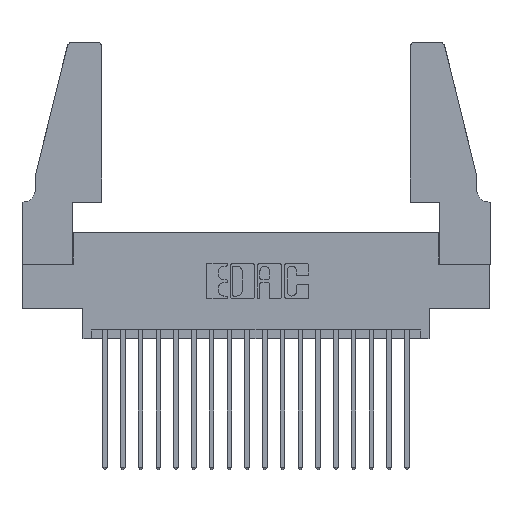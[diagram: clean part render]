
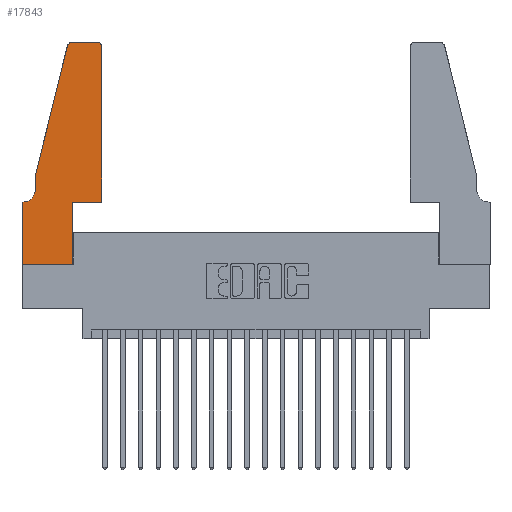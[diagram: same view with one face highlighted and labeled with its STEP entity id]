
A CAD part, top view. The second image highlights one B-rep face of the part: STEP entity #17843.
In plain terms, the highlighted planar face has unit normal (0, 0, 1).
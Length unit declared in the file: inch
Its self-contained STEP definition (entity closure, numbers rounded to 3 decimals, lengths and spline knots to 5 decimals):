
#2 = CARTESIAN_POINT ( 'NONE',  ( 0.0755, 0.5, 0.37 ) ) ;
#9 = DIRECTION ( 'NONE',  ( 0., 1., 0. ) ) ;
#520 = CARTESIAN_POINT ( 'NONE',  ( 0.4505, 0.35, 0.37 ) ) ;
#536 = ORIENTED_EDGE ( 'NONE', *, *, #3863, .T. ) ;
#631 = CARTESIAN_POINT ( 'NONE',  ( 0.4505, 0.35, 0.37 ) ) ;
#788 = DIRECTION ( 'NONE',  ( 0., 0., 1. ) ) ;
#1027 = LINE ( 'NONE', #520, #5373 ) ;
#1631 = VERTEX_POINT ( 'NONE', #18166 ) ;
#1721 = CARTESIAN_POINT ( 'NONE',  ( 0.0755, 0.42, 0.37 ) ) ;
#1843 = ORIENTED_EDGE ( 'NONE', *, *, #14942, .T. ) ;
#2127 = FACE_OUTER_BOUND ( 'NONE', #16101, .T. ) ;
#2367 = ORIENTED_EDGE ( 'NONE', *, *, #18949, .T. ) ;
#2944 = VERTEX_POINT ( 'NONE', #4091 ) ;
#3364 = VECTOR ( 'NONE', #5331, 39.37008 ) ;
#3475 = LINE ( 'NONE', #19083, #18404 ) ;
#3617 = EDGE_CURVE ( 'NONE', #4269, #6667, #7721, .T. ) ;
#3683 = DIRECTION ( 'NONE',  ( 0., 0., 1. ) ) ;
#3755 = CARTESIAN_POINT ( 'NONE',  ( 0.0755, 0.35, 0.37 ) ) ;
#3863 = EDGE_CURVE ( 'NONE', #18219, #6920, #7946, .T. ) ;
#3921 = ORIENTED_EDGE ( 'NONE', *, *, #6790, .T. ) ;
#3951 = EDGE_CURVE ( 'NONE', #12630, #5496, #13913, .T. ) ;
#4091 = CARTESIAN_POINT ( 'NONE',  ( 0.2865, 0.35, 0.37 ) ) ;
#4269 = VERTEX_POINT ( 'NONE', #14150 ) ;
#4566 = CARTESIAN_POINT ( 'NONE',  ( 0.4505, 1.22, 0.37 ) ) ;
#4882 = AXIS2_PLACEMENT_3D ( 'NONE', #5209, #3683, #14133 ) ;
#5209 = CARTESIAN_POINT ( 'NONE',  ( 0., 0.35, 0.37 ) ) ;
#5331 = DIRECTION ( 'NONE',  ( -1., 0., 0. ) ) ;
#5355 = LINE ( 'NONE', #2, #16715 ) ;
#5373 = VECTOR ( 'NONE', #11367, 39.37008 ) ;
#5496 = VERTEX_POINT ( 'NONE', #8089 ) ;
#5826 = EDGE_CURVE ( 'NONE', #6920, #4269, #3475, .T. ) ;
#6178 = AXIS2_PLACEMENT_3D ( 'NONE', #10851, #15654, #16074 ) ;
#6278 = CARTESIAN_POINT ( 'NONE',  ( 0., 0., 0.37 ) ) ;
#6507 = CARTESIAN_POINT ( 'NONE',  ( 0.0055, 0.42, 0.37 ) ) ;
#6520 = VERTEX_POINT ( 'NONE', #13166 ) ;
#6667 = VERTEX_POINT ( 'NONE', #7659 ) ;
#6790 = EDGE_CURVE ( 'NONE', #5496, #2944, #17440, .T. ) ;
#6920 = VERTEX_POINT ( 'NONE', #15602 ) ;
#7625 = CIRCLE ( 'NONE', #16728, 0.07 ) ;
#7659 = CARTESIAN_POINT ( 'NONE',  ( 0.25487, 1.22718, 0.37 ) ) ;
#7721 = CIRCLE ( 'NONE', #6178, 0.03 ) ;
#7946 = CIRCLE ( 'NONE', #16095, 0.03 ) ;
#8030 = DIRECTION ( 'NONE',  ( -1., 0., 0. ) ) ;
#8089 = CARTESIAN_POINT ( 'NONE',  ( 0.2865, 0., 0.37 ) ) ;
#8782 = DIRECTION ( 'NONE',  ( -1., 0., 0. ) ) ;
#9152 = ORIENTED_EDGE ( 'NONE', *, *, #5826, .T. ) ;
#9275 = CARTESIAN_POINT ( 'NONE',  ( 0.0055, 0.35, 0.37 ) ) ;
#10003 = DIRECTION ( 'NONE',  ( 0., 1., 0. ) ) ;
#10021 = VECTOR ( 'NONE', #19143, 39.37008 ) ;
#10087 = CARTESIAN_POINT ( 'NONE',  ( 0., 0., 0.37 ) ) ;
#10132 = CARTESIAN_POINT ( 'NONE',  ( 0.4205, 1.22, 0.37 ) ) ;
#10447 = EDGE_CURVE ( 'NONE', #17723, #12244, #7625, .T. ) ;
#10533 = ORIENTED_EDGE ( 'NONE', *, *, #10447, .T. ) ;
#10851 = CARTESIAN_POINT ( 'NONE',  ( 0.284, 1.22, 0.37 ) ) ;
#11367 = DIRECTION ( 'NONE',  ( 1., 0., 0. ) ) ;
#11447 = ORIENTED_EDGE ( 'NONE', *, *, #13132, .T. ) ;
#11605 = DIRECTION ( 'NONE',  ( 1., 0., 0. ) ) ;
#11637 = VECTOR ( 'NONE', #14301, 39.37008 ) ;
#11841 = LINE ( 'NONE', #3755, #3364 ) ;
#11903 = ORIENTED_EDGE ( 'NONE', *, *, #14478, .T. ) ;
#12244 = VERTEX_POINT ( 'NONE', #9275 ) ;
#12364 = DIRECTION ( 'NONE',  ( -0.239, -0.971, 0. ) ) ;
#12630 = VERTEX_POINT ( 'NONE', #10087 ) ;
#12641 = PLANE ( 'NONE',  #4882 ) ;
#13132 = EDGE_CURVE ( 'NONE', #6520, #12630, #17244, .T. ) ;
#13166 = CARTESIAN_POINT ( 'NONE',  ( 0., 0.35, 0.37 ) ) ;
#13504 = ORIENTED_EDGE ( 'NONE', *, *, #3617, .T. ) ;
#13505 = VECTOR ( 'NONE', #9, 39.37008 ) ;
#13913 = LINE ( 'NONE', #14534, #10021 ) ;
#14133 = DIRECTION ( 'NONE',  ( 1., 0., 0. ) ) ;
#14150 = CARTESIAN_POINT ( 'NONE',  ( 0.284, 1.25, 0.37 ) ) ;
#14301 = DIRECTION ( 'NONE',  ( 0., -1., 0. ) ) ;
#14409 = ORIENTED_EDGE ( 'NONE', *, *, #16006, .T. ) ;
#14478 = EDGE_CURVE ( 'NONE', #2944, #1631, #1027, .T. ) ;
#14534 = CARTESIAN_POINT ( 'NONE',  ( 0., 0., 0.37 ) ) ;
#14942 = EDGE_CURVE ( 'NONE', #6667, #18206, #5355, .T. ) ;
#14959 = CARTESIAN_POINT ( 'NONE',  ( 0.0755, 0.5, 0.37 ) ) ;
#15352 = ORIENTED_EDGE ( 'NONE', *, *, #3951, .T. ) ;
#15560 = LINE ( 'NONE', #631, #19480 ) ;
#15602 = CARTESIAN_POINT ( 'NONE',  ( 0.4205, 1.25, 0.37 ) ) ;
#15654 = DIRECTION ( 'NONE',  ( 0., 0., 1. ) ) ;
#15823 = ORIENTED_EDGE ( 'NONE', *, *, #19626, .T. ) ;
#16006 = EDGE_CURVE ( 'NONE', #12244, #6520, #11841, .T. ) ;
#16074 = DIRECTION ( 'NONE',  ( 1., 0., 0. ) ) ;
#16095 = AXIS2_PLACEMENT_3D ( 'NONE', #10132, #788, #11605 ) ;
#16101 = EDGE_LOOP ( 'NONE', ( #9152, #13504, #1843, #2367, #10533, #14409, #11447, #15352, #3921, #11903, #15823, #536 ) ) ;
#16715 = VECTOR ( 'NONE', #12364, 39.37008 ) ;
#16728 = AXIS2_PLACEMENT_3D ( 'NONE', #6507, #16847, #8030 ) ;
#16791 = VECTOR ( 'NONE', #18133, 39.37008 ) ;
#16847 = DIRECTION ( 'NONE',  ( 0., 0., -1. ) ) ;
#17244 = LINE ( 'NONE', #6278, #16791 ) ;
#17440 = LINE ( 'NONE', #18263, #13505 ) ;
#17723 = VERTEX_POINT ( 'NONE', #1721 ) ;
#17843 = ADVANCED_FACE ( 'NONE', ( #2127 ), #12641, .T. ) ;
#18133 = DIRECTION ( 'NONE',  ( 0., -1., 0. ) ) ;
#18166 = CARTESIAN_POINT ( 'NONE',  ( 0.4505, 0.35, 0.37 ) ) ;
#18206 = VERTEX_POINT ( 'NONE', #14959 ) ;
#18219 = VERTEX_POINT ( 'NONE', #4566 ) ;
#18263 = CARTESIAN_POINT ( 'NONE',  ( 0.2865, 0.35, 0.37 ) ) ;
#18404 = VECTOR ( 'NONE', #8782, 39.37008 ) ;
#18766 = CARTESIAN_POINT ( 'NONE',  ( 0.0755, 0.5, 0.37 ) ) ;
#18949 = EDGE_CURVE ( 'NONE', #18206, #17723, #19474, .T. ) ;
#19083 = CARTESIAN_POINT ( 'NONE',  ( 0.2605, 1.25, 0.37 ) ) ;
#19143 = DIRECTION ( 'NONE',  ( 1., 0., 0. ) ) ;
#19474 = LINE ( 'NONE', #18766, #11637 ) ;
#19480 = VECTOR ( 'NONE', #10003, 39.37008 ) ;
#19626 = EDGE_CURVE ( 'NONE', #1631, #18219, #15560, .T. ) ;
